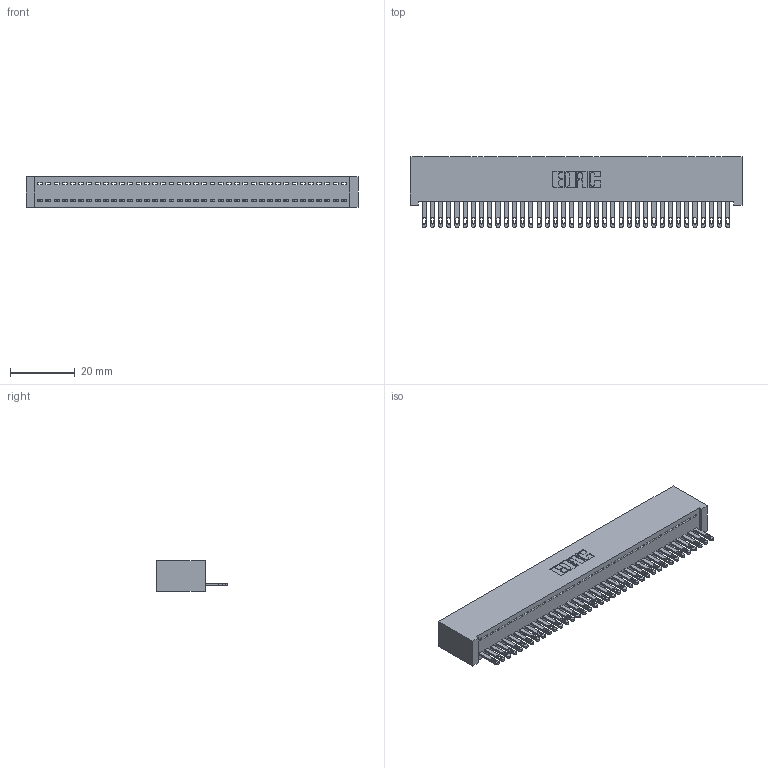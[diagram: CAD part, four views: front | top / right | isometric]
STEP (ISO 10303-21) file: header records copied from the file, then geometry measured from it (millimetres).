
FILE_DESCRIPTION (( 'STEP AP203' ), '1' );
FILE_NAME ('342-038-500-101.STEP', '2018-08-11T21:36:57', ( '' ), ( '' ), 'SwSTEP 2.0', 'SolidWorks 2016', '' );
FILE_SCHEMA (( 'CONFIG_CONTROL_DESIGN' ));
Length unit declared in the file: inch
Products named in the file (3): 342 Part_Lugless; 345-292-001_345-293-100; 342-038-500-101
Assembly tree (39 placements, depth 2):
  342-038-500-101
    342 Part_Lugless
    345-292-001_345-293-100  x38
Bounding box: 102.77 x 21.85 x 9.4 mm (x, y, z)
Volume: 9428.5 mm3; surface area: 14168.7 mm2
Topology: 39 solids, 39 shells, 2154 faces, 6659 edges, 4438 vertices
Faces by surface type: plane 1430, cylinder 724
Entity records: 23269 total; most frequent: CARTESIAN_POINT 4020, ORIENTED_EDGE 3994, DIRECTION 3393, EDGE_CURVE 1997, VECTOR 1873, LINE 1873, VERTEX_POINT 1330, AXIS2_PLACEMENT_3D 760
